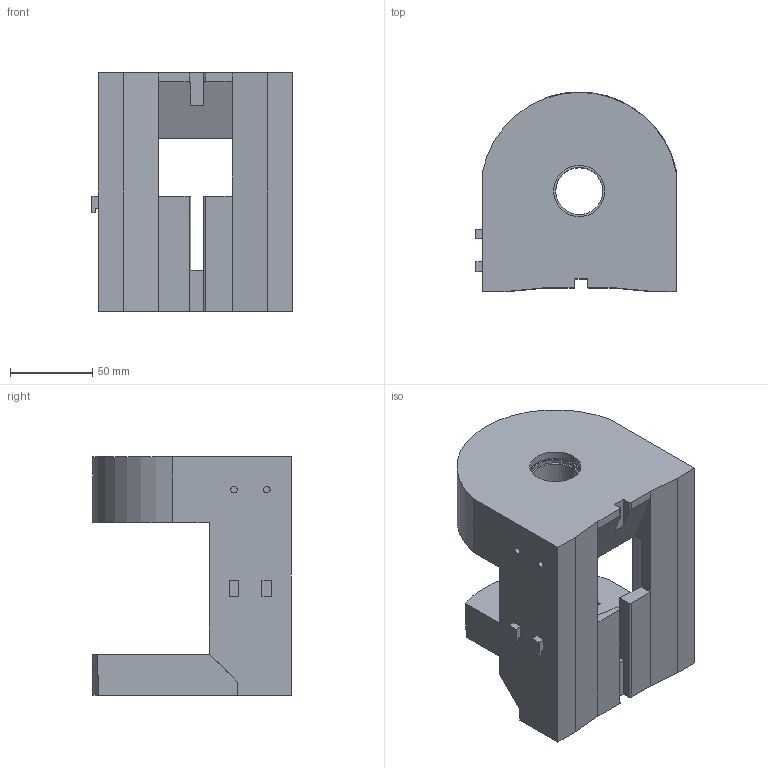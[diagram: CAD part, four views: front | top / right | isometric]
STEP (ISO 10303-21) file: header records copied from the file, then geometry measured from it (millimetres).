
FILE_DESCRIPTION (( 'STEP AP214' ), '1' );
FILE_NAME ('Reciver Exstention.STEP', '2025-05-18T11:16:52', ( '' ), ( '' ), 'SwSTEP 2.0', 'SolidWorks 2024', '' );
FILE_SCHEMA (( 'AUTOMOTIVE_DESIGN' ));
Length unit declared in the file: millimetre
Products named in the file (1): Reciver Exstention
Bounding box: 121.82 x 121 x 145 mm (x, y, z)
Volume: 850719.7 mm3; surface area: 106215.5 mm2
Topology: 1 solids, 1 shells, 115 faces, 307 edges, 202 vertices
Faces by surface type: plane 69, cylinder 42, cone 4
Entity records: 3704 total; most frequent: CARTESIAN_POINT 688, DIRECTION 634, ORIENTED_EDGE 614, EDGE_CURVE 307, AXIS2_PLACEMENT_3D 218, VERTEX_POINT 202, VECTOR 198, LINE 198
